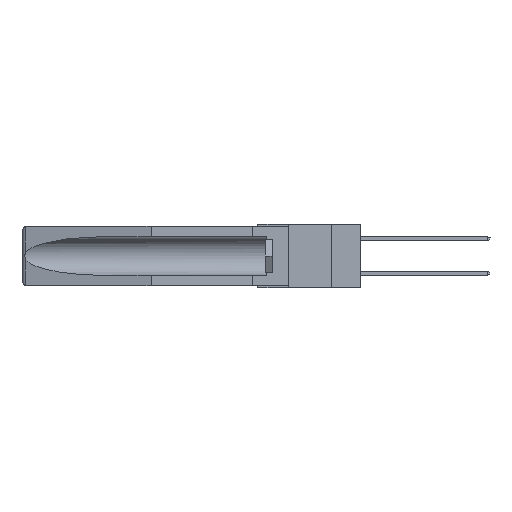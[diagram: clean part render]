
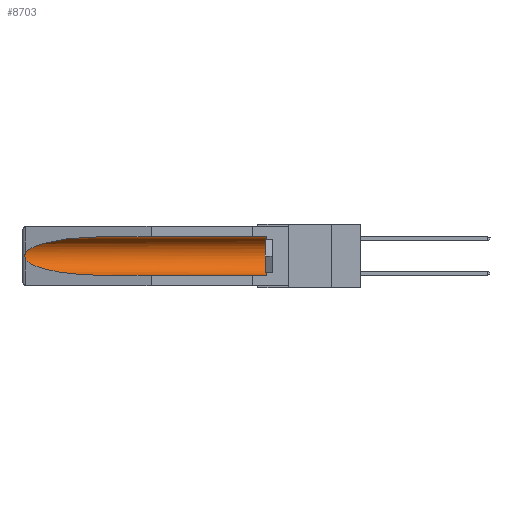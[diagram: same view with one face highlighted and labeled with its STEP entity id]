
A CAD part, left-side view. The second image highlights one B-rep face of the part: STEP entity #8703.
In plain terms, the highlighted cylindrical face has radius 2.857 mm (diameter 5.715 mm), a partial arc.
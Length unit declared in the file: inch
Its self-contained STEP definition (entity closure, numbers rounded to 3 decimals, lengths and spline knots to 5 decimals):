
#137 = CARTESIAN_POINT ( 'NONE',  ( 0.26537, 1.52718, -0.19328 ) ) ;
#369 = CARTESIAN_POINT ( 'NONE',  ( 0.2673, 1.53269, -0.17917 ) ) ;
#544 = CARTESIAN_POINT ( 'NONE',  ( 0.26537, 1.52718, -0.14972 ) ) ;
#829 = DIRECTION ( 'NONE',  ( 0., 1., 0. ) ) ;
#1121 = DIRECTION ( 'NONE',  ( 0., -1., 0. ) ) ;
#1281 = LINE ( 'NONE', #13910, #16948 ) ;
#1487 = CARTESIAN_POINT ( 'NONE',  ( 0.155, -0.30754, -0.1715 ) ) ;
#1974 = ORIENTED_EDGE ( 'NONE', *, *, #10807, .T. ) ;
#1977 =( BOUNDED_CURVE ( )  B_SPLINE_CURVE ( 3, ( #14050, #12448, #16853, #2308 ),
 .UNSPECIFIED., .F., .F. ) 
 B_SPLINE_CURVE_WITH_KNOTS ( ( 4, 4 ),
 ( 4.71239, 6.08839 ),
 .UNSPECIFIED. ) 
 CURVE ( )  GEOMETRIC_REPRESENTATION_ITEM ( )  RATIONAL_B_SPLINE_CURVE ( ( 1., 0.848, 0.848, 1. ) ) 
 REPRESENTATION_ITEM ( '' )  );
#1998 = EDGE_CURVE ( 'NONE', #15663, #6461, #1281, .T. ) ;
#2294 = CARTESIAN_POINT ( 'NONE',  ( 0.155, 0.126, -0.1715 ) ) ;
#2308 = CARTESIAN_POINT ( 'NONE',  ( 0.26537, 1.52718, -0.14972 ) ) ;
#2547 = ORIENTED_EDGE ( 'NONE', *, *, #4455, .F. ) ;
#2998 = LINE ( 'NONE', #9990, #17244 ) ;
#3034 = ORIENTED_EDGE ( 'NONE', *, *, #17666, .T. ) ;
#3064 = CARTESIAN_POINT ( 'NONE',  ( 0.25451, 1.48313, -0.24835 ) ) ;
#3421 = CARTESIAN_POINT ( 'NONE',  ( 0.2675, 1.53308, -0.17534 ) ) ;
#4360 = CARTESIAN_POINT ( 'NONE',  ( 0.21114, 1.30732, -0.284 ) ) ;
#4455 = EDGE_CURVE ( 'NONE', #16220, #12957, #2998, .T. ) ;
#4559 = CARTESIAN_POINT ( 'NONE',  ( 0.155, 1.07973, -0.284 ) ) ;
#4648 = EDGE_LOOP ( 'NONE', ( #10552, #3034, #1974, #2547, #9274, #17627 ) ) ;
#4949 = CARTESIAN_POINT ( 'NONE',  ( 0.26655, 1.53094, -0.18657 ) ) ;
#5352 = VERTEX_POINT ( 'NONE', #9922 ) ;
#6279 = CARTESIAN_POINT ( 'NONE',  ( 0.155, 0.126, -0.284 ) ) ;
#6461 = VERTEX_POINT ( 'NONE', #14001 ) ;
#6530 =( BOUNDED_CURVE ( )  B_SPLINE_CURVE ( 3, ( #14755, #3064, #4360, #4559 ),
 .UNSPECIFIED., .F., .F. ) 
 B_SPLINE_CURVE_WITH_KNOTS ( ( 4, 4 ),
 ( 0.1948, 1.5708 ),
 .UNSPECIFIED. ) 
 CURVE ( )  GEOMETRIC_REPRESENTATION_ITEM ( )  RATIONAL_B_SPLINE_CURVE ( ( 1., 0.848, 0.848, 1. ) ) 
 REPRESENTATION_ITEM ( '' )  );
#6614 = AXIS2_PLACEMENT_3D ( 'NONE', #2294, #1121, #8315 ) ;
#7516 = DIRECTION ( 'NONE',  ( 0., 1., 0. ) ) ;
#8315 = DIRECTION ( 'NONE',  ( 0., 0., 1. ) ) ;
#8703 = ADVANCED_FACE ( 'NONE', ( #17570 ), #14081, .F. ) ;
#9134 = CARTESIAN_POINT ( 'NONE',  ( 0.26597, 1.5296, -0.19026 ) ) ;
#9274 = ORIENTED_EDGE ( 'NONE', *, *, #13691, .T. ) ;
#9858 = VERTEX_POINT ( 'NONE', #137 ) ;
#9922 = CARTESIAN_POINT ( 'NONE',  ( 0.26537, 1.52718, -0.14972 ) ) ;
#9990 = CARTESIAN_POINT ( 'NONE',  ( 0.155, -0.30754, -0.284 ) ) ;
#10552 = ORIENTED_EDGE ( 'NONE', *, *, #11361, .T. ) ;
#10744 = CARTESIAN_POINT ( 'NONE',  ( 0.26597, 1.52961, -0.15275 ) ) ;
#10807 = EDGE_CURVE ( 'NONE', #9858, #12957, #6530, .T. ) ;
#11361 = EDGE_CURVE ( 'NONE', #6461, #5352, #1977, .T. ) ;
#12448 = CARTESIAN_POINT ( 'NONE',  ( 0.21114, 1.30732, -0.059 ) ) ;
#12957 = VERTEX_POINT ( 'NONE', #16717 ) ;
#13580 = CARTESIAN_POINT ( 'NONE',  ( 0.2673, 1.5327, -0.16383 ) ) ;
#13691 = EDGE_CURVE ( 'NONE', #16220, #15663, #16697, .T. ) ;
#13910 = CARTESIAN_POINT ( 'NONE',  ( 0.155, -0.30754, -0.059 ) ) ;
#14001 = CARTESIAN_POINT ( 'NONE',  ( 0.155, 1.07973, -0.059 ) ) ;
#14050 = CARTESIAN_POINT ( 'NONE',  ( 0.155, 1.07973, -0.059 ) ) ;
#14081 = CYLINDRICAL_SURFACE ( 'NONE', #14468, 0.1125 ) ;
#14468 = AXIS2_PLACEMENT_3D ( 'NONE', #1487, #7516, #16150 ) ;
#14755 = CARTESIAN_POINT ( 'NONE',  ( 0.26537, 1.52718, -0.19328 ) ) ;
#14942 = CARTESIAN_POINT ( 'NONE',  ( 0.155, 0.126, -0.059 ) ) ;
#15125 = CARTESIAN_POINT ( 'NONE',  ( 0.2675, 1.53308, -0.16763 ) ) ;
#15249 = CARTESIAN_POINT ( 'NONE',  ( 0.26654, 1.53092, -0.15636 ) ) ;
#15663 = VERTEX_POINT ( 'NONE', #14942 ) ;
#16150 = DIRECTION ( 'NONE',  ( 0., 0., 1. ) ) ;
#16206 = B_SPLINE_CURVE_WITH_KNOTS ( 'NONE', 3,
 ( #544, #10744, #15249, #13580, #15125, #3421, #369, #4949, #9134, #16676 ),
 .UNSPECIFIED., .F., .F.,
 ( 4, 2, 2, 2, 4 ),
 ( 0., 0.00029, 0.00058, 0.00087, 0.00117 ),
 .UNSPECIFIED. ) ;
#16220 = VERTEX_POINT ( 'NONE', #6279 ) ;
#16676 = CARTESIAN_POINT ( 'NONE',  ( 0.26537, 1.52718, -0.19328 ) ) ;
#16697 = CIRCLE ( 'NONE', #6614, 0.1125 ) ;
#16717 = CARTESIAN_POINT ( 'NONE',  ( 0.155, 1.07973, -0.284 ) ) ;
#16853 = CARTESIAN_POINT ( 'NONE',  ( 0.25451, 1.48313, -0.09465 ) ) ;
#16948 = VECTOR ( 'NONE', #829, 39.37008 ) ;
#17244 = VECTOR ( 'NONE', #17413, 39.37008 ) ;
#17413 = DIRECTION ( 'NONE',  ( 0., 1., 0. ) ) ;
#17570 = FACE_OUTER_BOUND ( 'NONE', #4648, .T. ) ;
#17627 = ORIENTED_EDGE ( 'NONE', *, *, #1998, .T. ) ;
#17666 = EDGE_CURVE ( 'NONE', #5352, #9858, #16206, .T. ) ;
